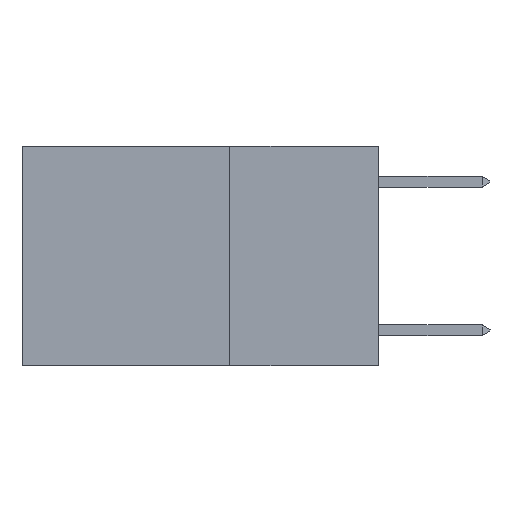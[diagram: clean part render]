
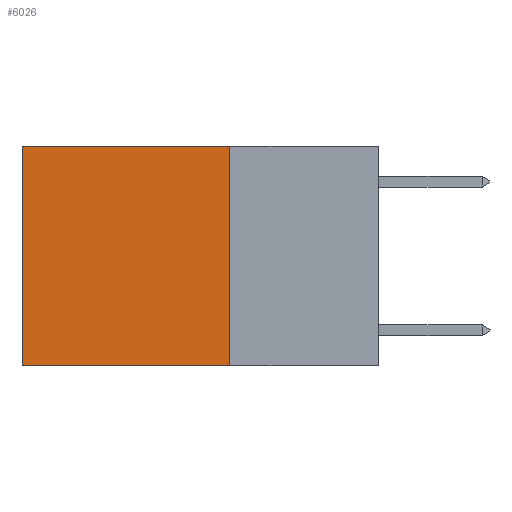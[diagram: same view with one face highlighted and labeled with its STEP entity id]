
A CAD part, left-side view. The second image highlights one B-rep face of the part: STEP entity #6026.
In plain terms, the highlighted planar face has unit normal (-1, 0, 0).
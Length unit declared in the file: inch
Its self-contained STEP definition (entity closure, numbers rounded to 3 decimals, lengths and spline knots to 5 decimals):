
#77 = EDGE_CURVE ( 'NONE', #273, #5637, #2163, .T. ) ;
#273 = VERTEX_POINT ( 'NONE', #864 ) ;
#864 = CARTESIAN_POINT ( 'NONE',  ( 0.2625, 0.6, 0. ) ) ;
#1331 = VERTEX_POINT ( 'NONE', #2816 ) ;
#1531 = CARTESIAN_POINT ( 'NONE',  ( 0.2625, 0.25, 0. ) ) ;
#1936 = CARTESIAN_POINT ( 'NONE',  ( 0.2625, 0.25, -0.37 ) ) ;
#1937 = ORIENTED_EDGE ( 'NONE', *, *, #9970, .T. ) ;
#2070 = DIRECTION ( 'NONE',  ( 0., 0., -1. ) ) ;
#2163 = LINE ( 'NONE', #11531, #9339 ) ;
#2403 = CARTESIAN_POINT ( 'NONE',  ( 0.2625, 0.25, 0. ) ) ;
#2816 = CARTESIAN_POINT ( 'NONE',  ( 0.2625, 0.25, 0. ) ) ;
#2879 = LINE ( 'NONE', #3573, #12538 ) ;
#3029 = VERTEX_POINT ( 'NONE', #1936 ) ;
#3457 = DIRECTION ( 'NONE',  ( 1., 0., 0. ) ) ;
#3542 = DIRECTION ( 'NONE',  ( 0., 1., 0. ) ) ;
#3573 = CARTESIAN_POINT ( 'NONE',  ( 0.2625, 0.25, 0. ) ) ;
#3641 = EDGE_CURVE ( 'NONE', #3029, #5637, #5358, .T. ) ;
#4540 = DIRECTION ( 'NONE',  ( 0., 0., -1. ) ) ;
#4832 = EDGE_CURVE ( 'NONE', #1331, #3029, #2879, .T. ) ;
#5358 = LINE ( 'NONE', #12496, #7588 ) ;
#5372 = ORIENTED_EDGE ( 'NONE', *, *, #4832, .F. ) ;
#5637 = VERTEX_POINT ( 'NONE', #8642 ) ;
#6026 = ADVANCED_FACE ( 'NONE', ( #11273 ), #8250, .F. ) ;
#6230 = EDGE_LOOP ( 'NONE', ( #8142, #11127, #5372, #1937 ) ) ;
#6464 = VECTOR ( 'NONE', #3542, 39.37008 ) ;
#7588 = VECTOR ( 'NONE', #9699, 39.37008 ) ;
#7797 = AXIS2_PLACEMENT_3D ( 'NONE', #2403, #3457, #10199 ) ;
#8142 = ORIENTED_EDGE ( 'NONE', *, *, #77, .T. ) ;
#8250 = PLANE ( 'NONE',  #7797 ) ;
#8642 = CARTESIAN_POINT ( 'NONE',  ( 0.2625, 0.6, -0.37 ) ) ;
#9339 = VECTOR ( 'NONE', #2070, 39.37008 ) ;
#9699 = DIRECTION ( 'NONE',  ( 0., 1., 0. ) ) ;
#9970 = EDGE_CURVE ( 'NONE', #1331, #273, #11341, .T. ) ;
#10199 = DIRECTION ( 'NONE',  ( 0., 0., -1. ) ) ;
#11127 = ORIENTED_EDGE ( 'NONE', *, *, #3641, .F. ) ;
#11273 = FACE_OUTER_BOUND ( 'NONE', #6230, .T. ) ;
#11341 = LINE ( 'NONE', #1531, #6464 ) ;
#11531 = CARTESIAN_POINT ( 'NONE',  ( 0.2625, 0.6, 0. ) ) ;
#12496 = CARTESIAN_POINT ( 'NONE',  ( 0.2625, 0.25, -0.37 ) ) ;
#12538 = VECTOR ( 'NONE', #4540, 39.37008 ) ;
